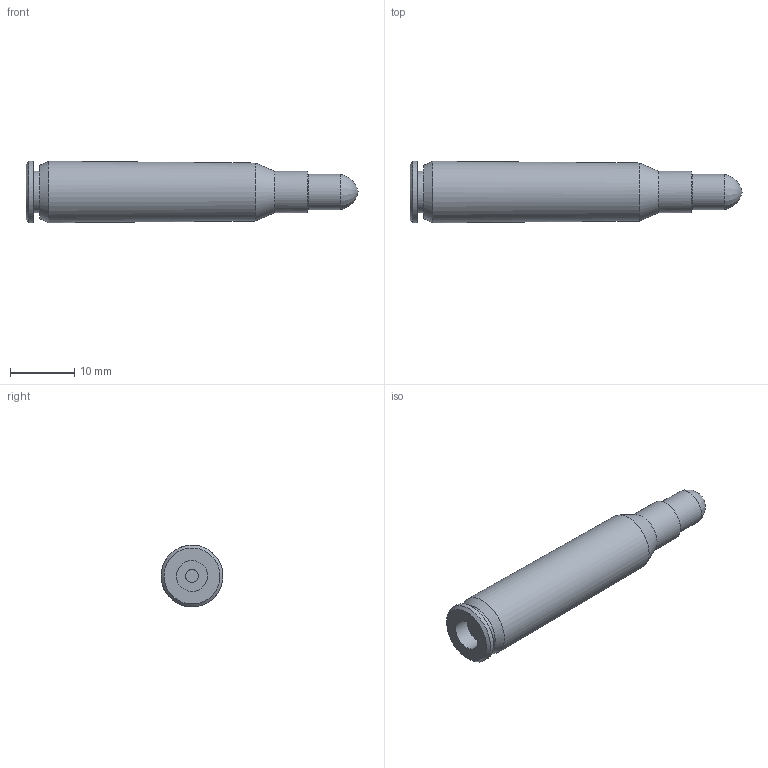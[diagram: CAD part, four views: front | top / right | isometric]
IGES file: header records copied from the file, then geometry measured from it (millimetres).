
Global section: file name: simunition .223 ammo referance v002; native system: Autodesk Inventor 2017; preprocessor: unknown; author: user; date: 20201115.154009; units: millimetre
Bounding box: 51.54 x 9.6 x 9.6 mm (x, y, z)
Volume: 1714.7 mm3; surface area: 4369.4 mm2
Topology: 5 solids, 5 shells, 81 faces, 218 edges, 153 vertices
Faces by surface type: bspline 81
